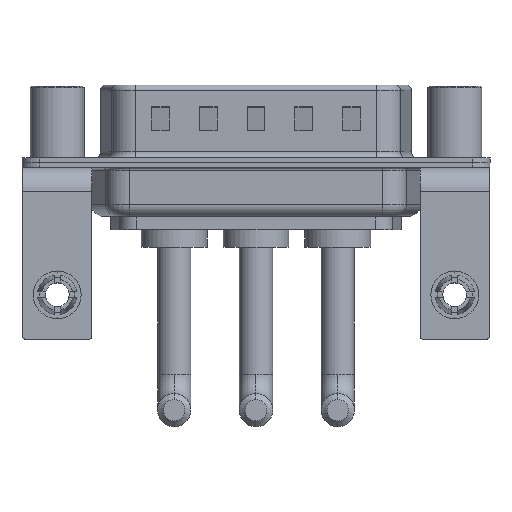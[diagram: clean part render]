
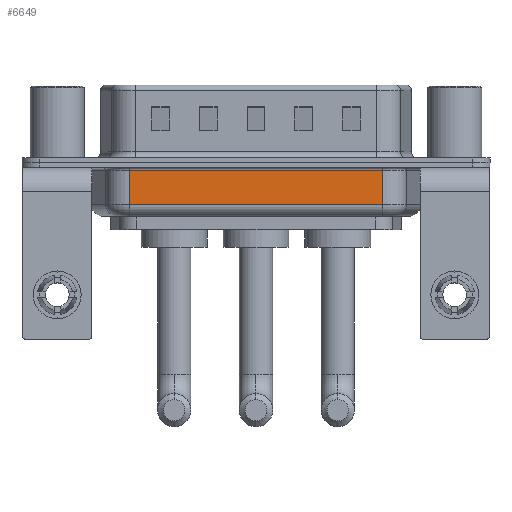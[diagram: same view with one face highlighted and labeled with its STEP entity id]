
A CAD part, front view. The second image highlights one B-rep face of the part: STEP entity #6649.
In plain terms, the highlighted planar face has unit normal (0, -1, 0).
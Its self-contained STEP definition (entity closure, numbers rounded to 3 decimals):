
#359 = CARTESIAN_POINT ( 'NONE',  ( 6.031, -5.35, -4.5 ) ) ;
#704 = ORIENTED_EDGE ( 'NONE', *, *, #10195, .T. ) ;
#1177 = DIRECTION ( 'NONE',  ( 0., 0., 1. ) ) ;
#2001 = EDGE_LOOP ( 'NONE', ( #11841, #704, #5820, #5940 ) ) ;
#2376 = VECTOR ( 'NONE', #4466, 1000. ) ;
#2682 = CARTESIAN_POINT ( 'NONE',  ( 27.269, -5.35, -4.5 ) ) ;
#4012 = EDGE_CURVE ( 'NONE', #9103, #12534, #12682, .T. ) ;
#4221 = VERTEX_POINT ( 'NONE', #5554 ) ;
#4259 = CARTESIAN_POINT ( 'NONE',  ( 6.031, -5.35, -3.5 ) ) ;
#4466 = DIRECTION ( 'NONE',  ( 1., 0., 0. ) ) ;
#4973 = VECTOR ( 'NONE', #15972, 1000. ) ;
#5554 = CARTESIAN_POINT ( 'NONE',  ( 27.269, -5.35, -3.5 ) ) ;
#5820 = ORIENTED_EDGE ( 'NONE', *, *, #11030, .T. ) ;
#5940 = ORIENTED_EDGE ( 'NONE', *, *, #10669, .T. ) ;
#6575 = VECTOR ( 'NONE', #1177, 1000. ) ;
#6649 = ADVANCED_FACE ( 'NONE', ( #16623 ), #9206, .F. ) ;
#7833 = VECTOR ( 'NONE', #12334, 1000. ) ;
#8568 = AXIS2_PLACEMENT_3D ( 'NONE', #15323, #18231, #16715 ) ;
#8760 = LINE ( 'NONE', #4259, #2376 ) ;
#8916 = CARTESIAN_POINT ( 'NONE',  ( 6.031, -5.35, -0.65 ) ) ;
#9103 = VERTEX_POINT ( 'NONE', #13148 ) ;
#9206 = PLANE ( 'NONE',  #8568 ) ;
#10195 = EDGE_CURVE ( 'NONE', #9103, #4221, #8760, .T. ) ;
#10669 = EDGE_CURVE ( 'NONE', #12372, #12534, #19756, .T. ) ;
#10735 = CARTESIAN_POINT ( 'NONE',  ( 27.269, -5.35, -0.65 ) ) ;
#11030 = EDGE_CURVE ( 'NONE', #4221, #12372, #16209, .T. ) ;
#11240 = CARTESIAN_POINT ( 'NONE',  ( 6.031, -5.35, -0.65 ) ) ;
#11841 = ORIENTED_EDGE ( 'NONE', *, *, #4012, .F. ) ;
#12334 = DIRECTION ( 'NONE',  ( -1., 0., 0. ) ) ;
#12372 = VERTEX_POINT ( 'NONE', #10735 ) ;
#12534 = VERTEX_POINT ( 'NONE', #11240 ) ;
#12682 = LINE ( 'NONE', #359, #4973 ) ;
#13148 = CARTESIAN_POINT ( 'NONE',  ( 6.031, -5.35, -3.5 ) ) ;
#15323 = CARTESIAN_POINT ( 'NONE',  ( 6.031, -5.35, -4.5 ) ) ;
#15972 = DIRECTION ( 'NONE',  ( 0., 0., 1. ) ) ;
#16209 = LINE ( 'NONE', #2682, #6575 ) ;
#16623 = FACE_OUTER_BOUND ( 'NONE', #2001, .T. ) ;
#16715 = DIRECTION ( 'NONE',  ( 0., 0., 1. ) ) ;
#18231 = DIRECTION ( 'NONE',  ( 0., 1., 0. ) ) ;
#19756 = LINE ( 'NONE', #8916, #7833 ) ;
